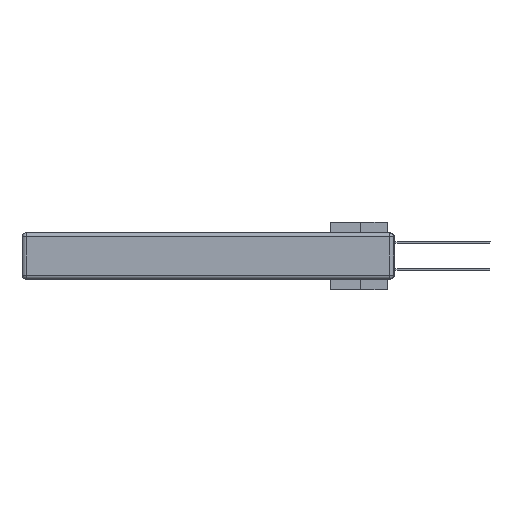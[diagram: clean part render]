
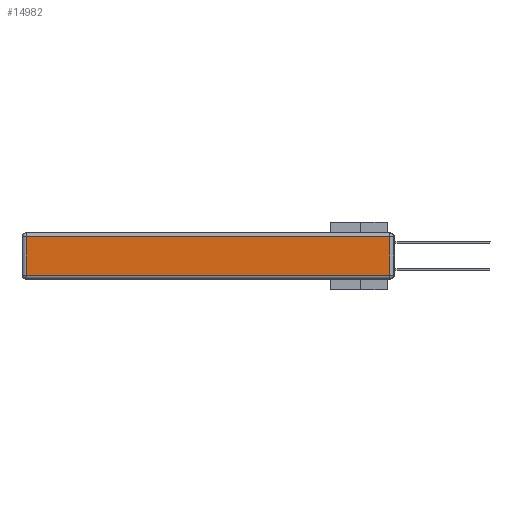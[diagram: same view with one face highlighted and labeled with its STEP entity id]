
A CAD part, left-side view. The second image highlights one B-rep face of the part: STEP entity #14982.
In plain terms, the highlighted planar face has unit normal (-1, 0, 0).
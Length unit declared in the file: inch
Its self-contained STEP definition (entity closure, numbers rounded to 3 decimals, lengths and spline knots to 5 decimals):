
#405 = CARTESIAN_POINT ( 'NONE',  ( 0., 2.72, -0.03 ) ) ;
#1321 = VERTEX_POINT ( 'NONE', #21608 ) ;
#2413 = CARTESIAN_POINT ( 'NONE',  ( 0., 0.03, -0.343 ) ) ;
#2771 = LINE ( 'NONE', #36397, #26519 ) ;
#2956 = CARTESIAN_POINT ( 'NONE',  ( 0., 2.75, -0.03 ) ) ;
#5218 = CARTESIAN_POINT ( 'NONE',  ( 0., 0., -0.343 ) ) ;
#5344 = EDGE_CURVE ( 'NONE', #32049, #29136, #2771, .T. ) ;
#6150 = ORIENTED_EDGE ( 'NONE', *, *, #26556, .T. ) ;
#8981 = AXIS2_PLACEMENT_3D ( 'NONE', #5218, #31731, #38280 ) ;
#10124 = CARTESIAN_POINT ( 'NONE',  ( 0., 0.03, -0.313 ) ) ;
#11184 = LINE ( 'NONE', #2413, #19911 ) ;
#11340 = LINE ( 'NONE', #32647, #32557 ) ;
#11583 = DIRECTION ( 'NONE',  ( 0., 0., 1. ) ) ;
#12367 = ORIENTED_EDGE ( 'NONE', *, *, #18475, .T. ) ;
#12965 = VECTOR ( 'NONE', #36002, 39.37008 ) ;
#13942 = DIRECTION ( 'NONE',  ( 0., 0., -1. ) ) ;
#14982 = ADVANCED_FACE ( 'NONE', ( #34905 ), #37882, .T. ) ;
#17509 = LINE ( 'NONE', #2956, #12965 ) ;
#18475 = EDGE_CURVE ( 'NONE', #21323, #32049, #11340, .T. ) ;
#19911 = VECTOR ( 'NONE', #11583, 39.37008 ) ;
#21323 = VERTEX_POINT ( 'NONE', #405 ) ;
#21608 = CARTESIAN_POINT ( 'NONE',  ( 0., 0.03, -0.03 ) ) ;
#25925 = EDGE_CURVE ( 'NONE', #1321, #21323, #17509, .T. ) ;
#26372 = ORIENTED_EDGE ( 'NONE', *, *, #5344, .T. ) ;
#26519 = VECTOR ( 'NONE', #30622, 39.37008 ) ;
#26556 = EDGE_CURVE ( 'NONE', #29136, #1321, #11184, .T. ) ;
#27065 = CARTESIAN_POINT ( 'NONE',  ( 0., 2.72, -0.313 ) ) ;
#28438 = ORIENTED_EDGE ( 'NONE', *, *, #25925, .T. ) ;
#29136 = VERTEX_POINT ( 'NONE', #10124 ) ;
#30622 = DIRECTION ( 'NONE',  ( 0., -1., 0. ) ) ;
#31731 = DIRECTION ( 'NONE',  ( -1., 0., 0. ) ) ;
#32049 = VERTEX_POINT ( 'NONE', #27065 ) ;
#32557 = VECTOR ( 'NONE', #13942, 39.37008 ) ;
#32647 = CARTESIAN_POINT ( 'NONE',  ( 0., 2.72, -0.343 ) ) ;
#33587 = EDGE_LOOP ( 'NONE', ( #26372, #6150, #28438, #12367 ) ) ;
#34905 = FACE_OUTER_BOUND ( 'NONE', #33587, .T. ) ;
#36002 = DIRECTION ( 'NONE',  ( 0., 1., 0. ) ) ;
#36397 = CARTESIAN_POINT ( 'NONE',  ( 0., 0., -0.313 ) ) ;
#37882 = PLANE ( 'NONE',  #8981 ) ;
#38280 = DIRECTION ( 'NONE',  ( 0., 0., 1. ) ) ;
